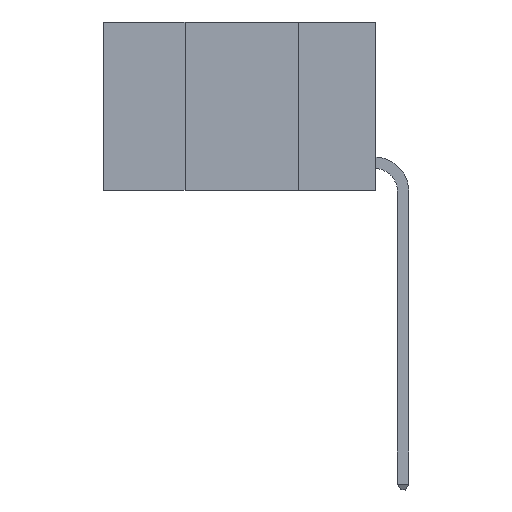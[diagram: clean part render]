
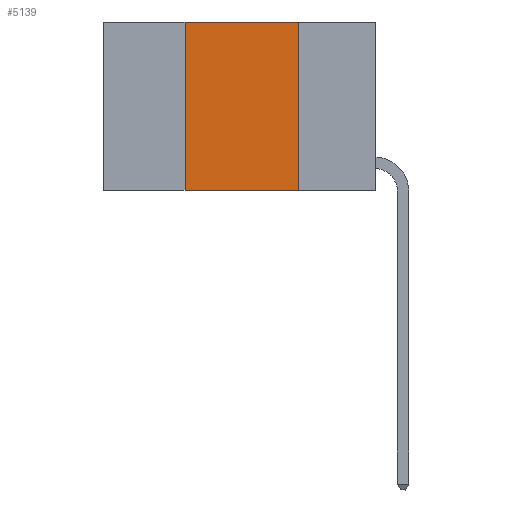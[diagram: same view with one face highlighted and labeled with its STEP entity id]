
A CAD part, left-side view. The second image highlights one B-rep face of the part: STEP entity #5139.
In plain terms, the highlighted planar face has unit normal (-1, 0, 0).
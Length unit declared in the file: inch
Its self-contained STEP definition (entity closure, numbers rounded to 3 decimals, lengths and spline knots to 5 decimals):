
#193 = LINE ( 'NONE', #12408, #23698 ) ;
#725 = VERTEX_POINT ( 'NONE', #19244 ) ;
#1538 = DIRECTION ( 'NONE',  ( 0., 0., 1. ) ) ;
#2733 = EDGE_CURVE ( 'NONE', #13719, #5061, #22261, .T. ) ;
#5061 = VERTEX_POINT ( 'NONE', #14867 ) ;
#5139 = ADVANCED_FACE ( 'NONE', ( #24973 ), #8322, .F. ) ;
#7658 = ORIENTED_EDGE ( 'NONE', *, *, #10567, .F. ) ;
#8322 = PLANE ( 'NONE',  #14966 ) ;
#10187 = VECTOR ( 'NONE', #16225, 39.37008 ) ;
#10567 = EDGE_CURVE ( 'NONE', #5061, #18678, #16217, .T. ) ;
#10617 = CARTESIAN_POINT ( 'NONE',  ( 0., 0.6, 0. ) ) ;
#10835 = DIRECTION ( 'NONE',  ( 0., -1., 0. ) ) ;
#11689 = CARTESIAN_POINT ( 'NONE',  ( 0., 0.6, 0. ) ) ;
#11927 = EDGE_CURVE ( 'NONE', #13719, #725, #26741, .T. ) ;
#12408 = CARTESIAN_POINT ( 'NONE',  ( 0., 0.17, 0. ) ) ;
#12905 = DIRECTION ( 'NONE',  ( 1., 0., 0. ) ) ;
#13719 = VERTEX_POINT ( 'NONE', #26559 ) ;
#14398 = ORIENTED_EDGE ( 'NONE', *, *, #11927, .T. ) ;
#14867 = CARTESIAN_POINT ( 'NONE',  ( 0., 0.42, 0. ) ) ;
#14966 = AXIS2_PLACEMENT_3D ( 'NONE', #10617, #12905, #28660 ) ;
#15436 = VECTOR ( 'NONE', #10835, 39.37008 ) ;
#16217 = LINE ( 'NONE', #11689, #10187 ) ;
#16225 = DIRECTION ( 'NONE',  ( 0., -1., 0. ) ) ;
#16240 = VECTOR ( 'NONE', #1538, 39.37008 ) ;
#18678 = VERTEX_POINT ( 'NONE', #26271 ) ;
#19244 = CARTESIAN_POINT ( 'NONE',  ( 0., 0.17, -0.37 ) ) ;
#22261 = LINE ( 'NONE', #28707, #16240 ) ;
#23698 = VECTOR ( 'NONE', #28177, 39.37008 ) ;
#24394 = CARTESIAN_POINT ( 'NONE',  ( 0., 0.6, -0.37 ) ) ;
#24973 = FACE_OUTER_BOUND ( 'NONE', #26332, .T. ) ;
#25002 = ORIENTED_EDGE ( 'NONE', *, *, #26096, .F. ) ;
#25701 = ORIENTED_EDGE ( 'NONE', *, *, #2733, .F. ) ;
#26096 = EDGE_CURVE ( 'NONE', #18678, #725, #193, .T. ) ;
#26271 = CARTESIAN_POINT ( 'NONE',  ( 0., 0.17, 0. ) ) ;
#26332 = EDGE_LOOP ( 'NONE', ( #25002, #7658, #25701, #14398 ) ) ;
#26559 = CARTESIAN_POINT ( 'NONE',  ( 0., 0.42, -0.37 ) ) ;
#26741 = LINE ( 'NONE', #24394, #15436 ) ;
#28177 = DIRECTION ( 'NONE',  ( 0., 0., -1. ) ) ;
#28660 = DIRECTION ( 'NONE',  ( 0., 0., -1. ) ) ;
#28707 = CARTESIAN_POINT ( 'NONE',  ( 0., 0.42, 0. ) ) ;
